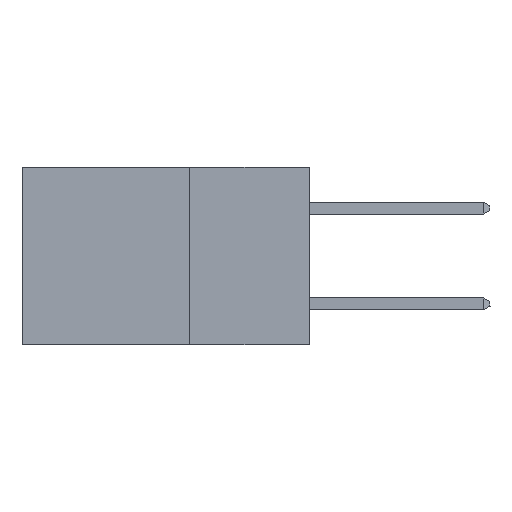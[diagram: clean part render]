
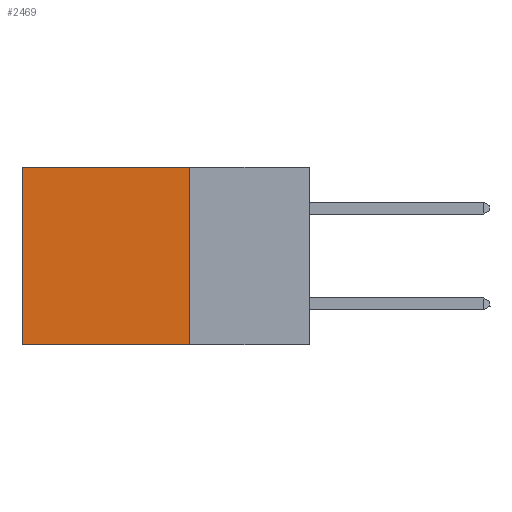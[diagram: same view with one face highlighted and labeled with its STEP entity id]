
A CAD part, left-side view. The second image highlights one B-rep face of the part: STEP entity #2469.
In plain terms, the highlighted planar face has unit normal (-1, 0, 0).
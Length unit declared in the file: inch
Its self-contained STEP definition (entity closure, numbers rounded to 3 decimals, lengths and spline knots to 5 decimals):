
#234 = CARTESIAN_POINT ( 'NONE',  ( 0.2875, 0.25, 0. ) ) ;
#542 = EDGE_CURVE ( 'NONE', #27234, #3623, #10044, .T. ) ;
#656 = DIRECTION ( 'NONE',  ( 0., 1., 0. ) ) ;
#752 = CARTESIAN_POINT ( 'NONE',  ( 0.2875, 0.25, -0.37 ) ) ;
#1948 = CARTESIAN_POINT ( 'NONE',  ( 0.2875, 0.6, 0. ) ) ;
#2019 = AXIS2_PLACEMENT_3D ( 'NONE', #234, #11556, #17960 ) ;
#2469 = ADVANCED_FACE ( 'NONE', ( #7796 ), #4682, .F. ) ;
#3623 = VERTEX_POINT ( 'NONE', #1948 ) ;
#3978 = ORIENTED_EDGE ( 'NONE', *, *, #12529, .F. ) ;
#4660 = EDGE_LOOP ( 'NONE', ( #20875, #3978, #17449, #28130 ) ) ;
#4682 = PLANE ( 'NONE',  #2019 ) ;
#6239 = CARTESIAN_POINT ( 'NONE',  ( 0.2875, 0.25, 0. ) ) ;
#6243 = EDGE_CURVE ( 'NONE', #27234, #26173, #11044, .T. ) ;
#6995 = LINE ( 'NONE', #752, #18611 ) ;
#7024 = DIRECTION ( 'NONE',  ( 0., 0., -1. ) ) ;
#7796 = FACE_OUTER_BOUND ( 'NONE', #4660, .T. ) ;
#8003 = DIRECTION ( 'NONE',  ( 0., 0., -1. ) ) ;
#10044 = LINE ( 'NONE', #6239, #24459 ) ;
#10345 = VECTOR ( 'NONE', #8003, 39.37008 ) ;
#10973 = EDGE_CURVE ( 'NONE', #3623, #11314, #24301, .T. ) ;
#11044 = LINE ( 'NONE', #16882, #10345 ) ;
#11314 = VERTEX_POINT ( 'NONE', #12496 ) ;
#11556 = DIRECTION ( 'NONE',  ( 1., 0., 0. ) ) ;
#12496 = CARTESIAN_POINT ( 'NONE',  ( 0.2875, 0.6, -0.37 ) ) ;
#12529 = EDGE_CURVE ( 'NONE', #26173, #11314, #6995, .T. ) ;
#16598 = VECTOR ( 'NONE', #7024, 39.37008 ) ;
#16882 = CARTESIAN_POINT ( 'NONE',  ( 0.2875, 0.25, 0. ) ) ;
#17449 = ORIENTED_EDGE ( 'NONE', *, *, #6243, .F. ) ;
#17960 = DIRECTION ( 'NONE',  ( 0., 0., -1. ) ) ;
#18611 = VECTOR ( 'NONE', #656, 39.37008 ) ;
#20475 = CARTESIAN_POINT ( 'NONE',  ( 0.2875, 0.6, 0. ) ) ;
#20875 = ORIENTED_EDGE ( 'NONE', *, *, #10973, .T. ) ;
#24301 = LINE ( 'NONE', #20475, #16598 ) ;
#24459 = VECTOR ( 'NONE', #28740, 39.37008 ) ;
#25846 = CARTESIAN_POINT ( 'NONE',  ( 0.2875, 0.25, -0.37 ) ) ;
#26173 = VERTEX_POINT ( 'NONE', #25846 ) ;
#27142 = CARTESIAN_POINT ( 'NONE',  ( 0.2875, 0.25, 0. ) ) ;
#27234 = VERTEX_POINT ( 'NONE', #27142 ) ;
#28130 = ORIENTED_EDGE ( 'NONE', *, *, #542, .T. ) ;
#28740 = DIRECTION ( 'NONE',  ( 0., 1., 0. ) ) ;
